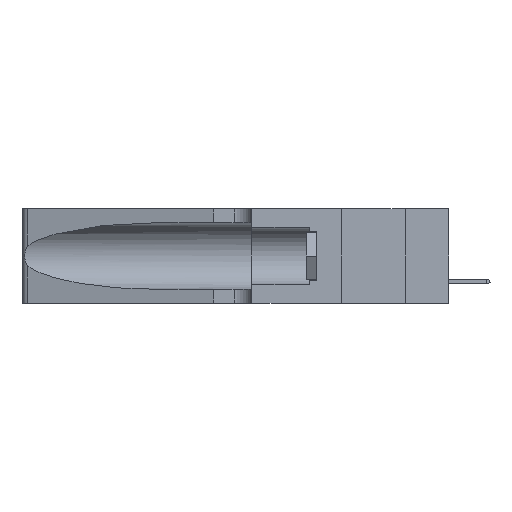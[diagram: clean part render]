
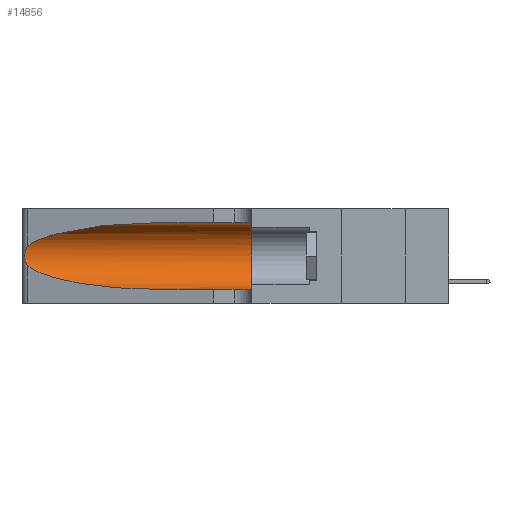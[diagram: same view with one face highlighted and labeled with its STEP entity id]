
A CAD part, left-side view. The second image highlights one B-rep face of the part: STEP entity #14856.
In plain terms, the highlighted cylindrical face has radius 3.308 mm (diameter 6.617 mm), a partial arc.
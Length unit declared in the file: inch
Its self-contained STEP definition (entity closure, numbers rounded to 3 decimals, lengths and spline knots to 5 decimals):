
#397 = AXIS2_PLACEMENT_3D ( 'NONE', #572, #6412, #2505 ) ;
#483 = ORIENTED_EDGE ( 'NONE', *, *, #6537, .F. ) ;
#572 = CARTESIAN_POINT ( 'NONE',  ( 0.1305, 1.61858, 0.185 ) ) ;
#1653 = CARTESIAN_POINT ( 'NONE',  ( 0.25487, 1.22718, 0.22369 ) ) ;
#1731 = CARTESIAN_POINT ( 'NONE',  ( 0.25555, 1.22994, 0.2215 ) ) ;
#1898 = VERTEX_POINT ( 'NONE', #2361 ) ;
#2336 = ORIENTED_EDGE ( 'NONE', *, *, #15259, .T. ) ;
#2361 = CARTESIAN_POINT ( 'NONE',  ( 0.1305, 0.72297, 0.05475 ) ) ;
#2505 = DIRECTION ( 'NONE',  ( 0., 0., -1. ) ) ;
#2897 = EDGE_CURVE ( 'NONE', #18562, #7818, #14887, .T. ) ;
#3499 = CARTESIAN_POINT ( 'NONE',  ( 0.26018, 1.23835, 0.19895 ) ) ;
#3581 = CARTESIAN_POINT ( 'NONE',  ( 0.26075, 1.23896, 0.178 ) ) ;
#3638 = CARTESIAN_POINT ( 'NONE',  ( 0.18966, 0.96281, 0.05475 ) ) ;
#4649 = EDGE_CURVE ( 'NONE', #18562, #6149, #17460, .T. ) ;
#5165 = EDGE_CURVE ( 'NONE', #1898, #12917, #22759, .T. ) ;
#6149 = VERTEX_POINT ( 'NONE', #13391 ) ;
#6412 = DIRECTION ( 'NONE',  ( 0., -1., 0. ) ) ;
#6537 = EDGE_CURVE ( 'NONE', #7818, #12917, #17076, .T. ) ;
#7243 = CARTESIAN_POINT ( 'NONE',  ( 0.18966, 0.96281, 0.31525 ) ) ;
#7330 = CARTESIAN_POINT ( 'NONE',  ( 0.25856, 1.23593, 0.16098 ) ) ;
#7818 = VERTEX_POINT ( 'NONE', #19444 ) ;
#7904 = DIRECTION ( 'NONE',  ( 0., -1., 0. ) ) ;
#9209 = CARTESIAN_POINT ( 'NONE',  ( 0.25555, 1.22993, 0.14849 ) ) ;
#9841 = CARTESIAN_POINT ( 'NONE',  ( 0.25487, 1.22718, 0.22369 ) ) ;
#10307 = CARTESIAN_POINT ( 'NONE',  ( 0.1305, 1.61858, 0.05475 ) ) ;
#10792 = DIRECTION ( 'NONE',  ( 0., -1., 0. ) ) ;
#12470 = CARTESIAN_POINT ( 'NONE',  ( 0.1305, 0.72297, 0.31525 ) ) ;
#12917 = VERTEX_POINT ( 'NONE', #16148 ) ;
#12996 = CARTESIAN_POINT ( 'NONE',  ( 0.25854, 1.2359, 0.20912 ) ) ;
#13146 = CARTESIAN_POINT ( 'NONE',  ( 0.1305, 0.72297, 0.31525 ) ) ;
#13246 = DIRECTION ( 'NONE',  ( 0., 0., 1. ) ) ;
#13391 = CARTESIAN_POINT ( 'NONE',  ( 0.25487, 1.22718, 0.22369 ) ) ;
#13500 = CARTESIAN_POINT ( 'NONE',  ( 0.1305, 0.35, 0.185 ) ) ;
#13523 = VECTOR ( 'NONE', #10792, 39.37008 ) ;
#13952 = ORIENTED_EDGE ( 'NONE', *, *, #5165, .T. ) ;
#14856 = ADVANCED_FACE ( 'NONE', ( #24019 ), #15068, .F. ) ;
#14887 = LINE ( 'NONE', #17596, #20243 ) ;
#14900 = CARTESIAN_POINT ( 'NONE',  ( 0.25787, 1.23484, 0.2124 ) ) ;
#15065 = CARTESIAN_POINT ( 'NONE',  ( 0.25789, 1.23486, 0.15765 ) ) ;
#15068 = CYLINDRICAL_SURFACE ( 'NONE', #397, 0.13025 ) ;
#15123 = CARTESIAN_POINT ( 'NONE',  ( 0.1305, 0.72297, 0.05475 ) ) ;
#15259 = EDGE_CURVE ( 'NONE', #6149, #17175, #21100, .T. ) ;
#15418 = AXIS2_PLACEMENT_3D ( 'NONE', #13500, #24685, #13246 ) ;
#15457 = CARTESIAN_POINT ( 'NONE',  ( 0.25487, 1.22718, 0.14631 ) ) ;
#15929 =( BOUNDED_CURVE ( )  B_SPLINE_CURVE ( 3, ( #22854, #22613, #3638, #15123 ),
 .UNSPECIFIED., .F., .T. ) 
 B_SPLINE_CURVE_WITH_KNOTS ( ( 4, 4 ),
 ( 3.44316, 4.71239 ),
 .UNSPECIFIED. ) 
 CURVE ( )  GEOMETRIC_REPRESENTATION_ITEM ( )  RATIONAL_B_SPLINE_CURVE ( ( 1., 0.87, 0.87, 1. ) ) 
 REPRESENTATION_ITEM ( '' )  );
#16148 = CARTESIAN_POINT ( 'NONE',  ( 0.1305, 0.35, 0.05475 ) ) ;
#16757 = CARTESIAN_POINT ( 'NONE',  ( 0.2373, 1.15595, 0.28018 ) ) ;
#16847 = CARTESIAN_POINT ( 'NONE',  ( 0.26075, 1.23896, 0.19203 ) ) ;
#17076 = CIRCLE ( 'NONE', #15418, 0.13025 ) ;
#17175 = VERTEX_POINT ( 'NONE', #15457 ) ;
#17460 =( BOUNDED_CURVE ( )  B_SPLINE_CURVE ( 3, ( #13146, #7243, #16757, #9841 ),
 .UNSPECIFIED., .F., .F. ) 
 B_SPLINE_CURVE_WITH_KNOTS ( ( 4, 4 ),
 ( 1.5708, 2.84003 ),
 .UNSPECIFIED. ) 
 CURVE ( )  GEOMETRIC_REPRESENTATION_ITEM ( )  RATIONAL_B_SPLINE_CURVE ( ( 1., 0.87, 0.87, 1. ) ) 
 REPRESENTATION_ITEM ( '' )  );
#17596 = CARTESIAN_POINT ( 'NONE',  ( 0.1305, 1.61858, 0.31525 ) ) ;
#18562 = VERTEX_POINT ( 'NONE', #12470 ) ;
#18727 = CARTESIAN_POINT ( 'NONE',  ( 0.26017, 1.23833, 0.17102 ) ) ;
#18889 = CARTESIAN_POINT ( 'NONE',  ( 0.25487, 1.22718, 0.14631 ) ) ;
#19133 = EDGE_LOOP ( 'NONE', ( #24727, #2336, #23810, #13952, #483, #22923 ) ) ;
#19444 = CARTESIAN_POINT ( 'NONE',  ( 0.1305, 0.35, 0.31525 ) ) ;
#20243 = VECTOR ( 'NONE', #7904, 39.37008 ) ;
#20652 = CARTESIAN_POINT ( 'NONE',  ( 0.25639, 1.23186, 0.15144 ) ) ;
#21100 = B_SPLINE_CURVE_WITH_KNOTS ( 'NONE', 3,
 ( #1653, #1731, #24414, #14900, #12996, #3499, #16847, #3581, #18727, #7330, #15065, #20652, #9209, #18889 ),
 .UNSPECIFIED., .F., .F.,
 ( 4, 2, 2, 2, 2, 2, 4 ),
 ( 0., 0.00027, 0.00053, 0.00107, 0.0016, 0.00187, 0.00214 ),
 .UNSPECIFIED. ) ;
#21677 = EDGE_CURVE ( 'NONE', #17175, #1898, #15929, .T. ) ;
#22613 = CARTESIAN_POINT ( 'NONE',  ( 0.2373, 1.15595, 0.08982 ) ) ;
#22759 = LINE ( 'NONE', #10307, #13523 ) ;
#22854 = CARTESIAN_POINT ( 'NONE',  ( 0.25487, 1.22718, 0.14631 ) ) ;
#22923 = ORIENTED_EDGE ( 'NONE', *, *, #2897, .F. ) ;
#23810 = ORIENTED_EDGE ( 'NONE', *, *, #21677, .T. ) ;
#24019 = FACE_OUTER_BOUND ( 'NONE', #19133, .T. ) ;
#24414 = CARTESIAN_POINT ( 'NONE',  ( 0.25639, 1.23184, 0.21858 ) ) ;
#24685 = DIRECTION ( 'NONE',  ( 0., 1., 0. ) ) ;
#24727 = ORIENTED_EDGE ( 'NONE', *, *, #4649, .T. ) ;
